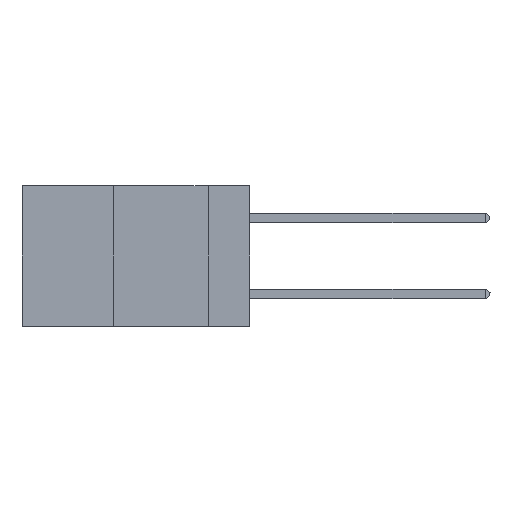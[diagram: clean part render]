
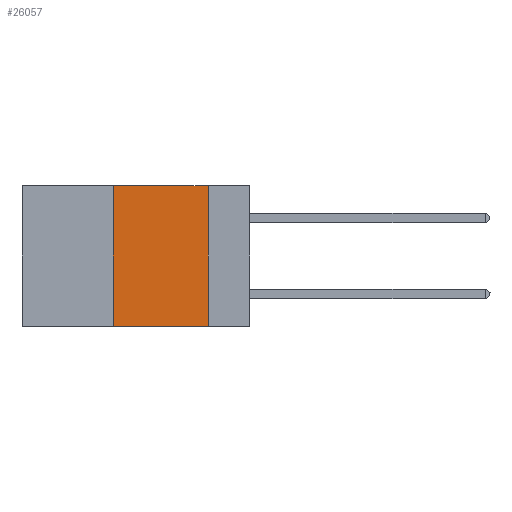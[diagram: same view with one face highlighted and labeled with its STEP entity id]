
A CAD part, left-side view. The second image highlights one B-rep face of the part: STEP entity #26057.
In plain terms, the highlighted planar face has unit normal (-1, 0, 0).
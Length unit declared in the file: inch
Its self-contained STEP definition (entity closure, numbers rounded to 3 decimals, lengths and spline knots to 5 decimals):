
#254 = CARTESIAN_POINT ( 'NONE',  ( 0., 0.11, -0.37 ) ) ;
#373 = CARTESIAN_POINT ( 'NONE',  ( 0., 0.11, 0. ) ) ;
#1370 = VECTOR ( 'NONE', #17295, 39.37008 ) ;
#2670 = LINE ( 'NONE', #373, #18197 ) ;
#2890 = VERTEX_POINT ( 'NONE', #16461 ) ;
#8217 = DIRECTION ( 'NONE',  ( 0., -1., 0. ) ) ;
#8274 = VECTOR ( 'NONE', #22199, 39.37008 ) ;
#8359 = AXIS2_PLACEMENT_3D ( 'NONE', #24606, #9399, #26093 ) ;
#8423 = LINE ( 'NONE', #10711, #1370 ) ;
#9399 = DIRECTION ( 'NONE',  ( 1., 0., 0. ) ) ;
#10084 = CARTESIAN_POINT ( 'NONE',  ( 0., 0.11, 0. ) ) ;
#10711 = CARTESIAN_POINT ( 'NONE',  ( 0., 0.6, 0. ) ) ;
#11841 = FACE_OUTER_BOUND ( 'NONE', #13904, .T. ) ;
#12931 = ORIENTED_EDGE ( 'NONE', *, *, #23396, .F. ) ;
#13393 = ORIENTED_EDGE ( 'NONE', *, *, #24225, .F. ) ;
#13462 = ORIENTED_EDGE ( 'NONE', *, *, #14364, .F. ) ;
#13904 = EDGE_LOOP ( 'NONE', ( #13462, #12931, #13393, #18706 ) ) ;
#14364 = EDGE_CURVE ( 'NONE', #16827, #19103, #2670, .T. ) ;
#14938 = CARTESIAN_POINT ( 'NONE',  ( 0., 0.6, -0.37 ) ) ;
#16461 = CARTESIAN_POINT ( 'NONE',  ( 0., 0.36, 0. ) ) ;
#16827 = VERTEX_POINT ( 'NONE', #10084 ) ;
#17295 = DIRECTION ( 'NONE',  ( 0., -1., 0. ) ) ;
#17330 = PLANE ( 'NONE',  #8359 ) ;
#18197 = VECTOR ( 'NONE', #21754, 39.37008 ) ;
#18706 = ORIENTED_EDGE ( 'NONE', *, *, #26700, .T. ) ;
#19103 = VERTEX_POINT ( 'NONE', #254 ) ;
#20462 = LINE ( 'NONE', #27081, #8274 ) ;
#21754 = DIRECTION ( 'NONE',  ( 0., 0., -1. ) ) ;
#22199 = DIRECTION ( 'NONE',  ( 0., 0., 1. ) ) ;
#23396 = EDGE_CURVE ( 'NONE', #2890, #16827, #8423, .T. ) ;
#23427 = LINE ( 'NONE', #14938, #25305 ) ;
#24225 = EDGE_CURVE ( 'NONE', #25121, #2890, #20462, .T. ) ;
#24414 = CARTESIAN_POINT ( 'NONE',  ( 0., 0.36, -0.37 ) ) ;
#24606 = CARTESIAN_POINT ( 'NONE',  ( 0., 0.6, 0. ) ) ;
#25121 = VERTEX_POINT ( 'NONE', #24414 ) ;
#25305 = VECTOR ( 'NONE', #8217, 39.37008 ) ;
#26057 = ADVANCED_FACE ( 'NONE', ( #11841 ), #17330, .F. ) ;
#26093 = DIRECTION ( 'NONE',  ( 0., 0., -1. ) ) ;
#26700 = EDGE_CURVE ( 'NONE', #25121, #19103, #23427, .T. ) ;
#27081 = CARTESIAN_POINT ( 'NONE',  ( 0., 0.36, 0. ) ) ;
